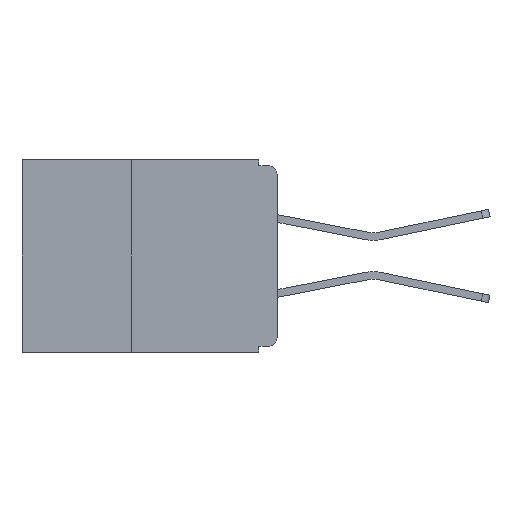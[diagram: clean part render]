
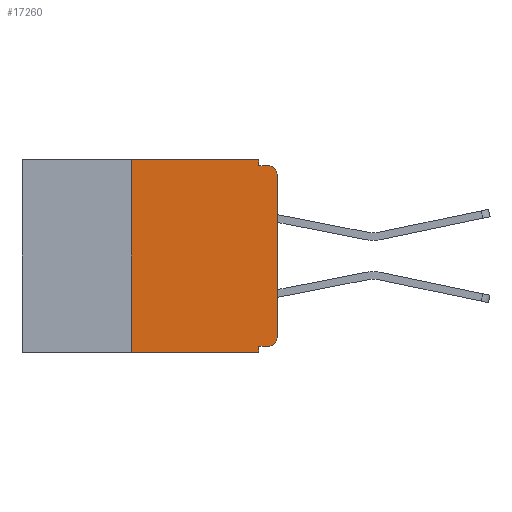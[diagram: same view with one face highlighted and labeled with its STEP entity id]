
A CAD part, left-side view. The second image highlights one B-rep face of the part: STEP entity #17260.
In plain terms, the highlighted planar face has unit normal (-1, 0, 0).
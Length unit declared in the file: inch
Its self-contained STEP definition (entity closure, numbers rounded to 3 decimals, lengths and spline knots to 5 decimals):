
#259 = CARTESIAN_POINT ( 'NONE',  ( 0., 0., -0.305 ) ) ;
#362 = CARTESIAN_POINT ( 'NONE',  ( 0., 0.015, -0.305 ) ) ;
#525 = LINE ( 'NONE', #21189, #6271 ) ;
#812 = CIRCLE ( 'NONE', #27295, 0.015 ) ;
#1344 = ORIENTED_EDGE ( 'NONE', *, *, #1648, .F. ) ;
#1469 = ORIENTED_EDGE ( 'NONE', *, *, #7640, .F. ) ;
#1493 = AXIS2_PLACEMENT_3D ( 'NONE', #25879, #11175, #28337 ) ;
#1648 = EDGE_CURVE ( 'NONE', #16640, #24566, #22728, .T. ) ;
#1978 = EDGE_CURVE ( 'NONE', #24566, #7987, #525, .T. ) ;
#2116 = CARTESIAN_POINT ( 'NONE',  ( 0., 0.25, -0.33 ) ) ;
#2266 = DIRECTION ( 'NONE',  ( 0., 0., -1. ) ) ;
#2871 = DIRECTION ( 'NONE',  ( 0., 0., -1. ) ) ;
#3144 = LINE ( 'NONE', #5762, #28352 ) ;
#4116 = CARTESIAN_POINT ( 'NONE',  ( 0., 0.25, 0. ) ) ;
#5068 = ORIENTED_EDGE ( 'NONE', *, *, #12646, .T. ) ;
#5255 = VERTEX_POINT ( 'NONE', #22413 ) ;
#5286 = VECTOR ( 'NONE', #30228, 39.37008 ) ;
#5336 = ORIENTED_EDGE ( 'NONE', *, *, #23204, .F. ) ;
#5560 = CARTESIAN_POINT ( 'NONE',  ( 0., 0.031, 0. ) ) ;
#5762 = CARTESIAN_POINT ( 'NONE',  ( 0., 0.437, -0.33 ) ) ;
#6271 = VECTOR ( 'NONE', #25772, 39.37008 ) ;
#7194 = CARTESIAN_POINT ( 'NONE',  ( 0., 0., -0.025 ) ) ;
#7640 = EDGE_CURVE ( 'NONE', #5255, #25740, #27625, .T. ) ;
#7987 = VERTEX_POINT ( 'NONE', #16604 ) ;
#8004 = DIRECTION ( 'NONE',  ( 0., -1., 0. ) ) ;
#8233 = ORIENTED_EDGE ( 'NONE', *, *, #10776, .F. ) ;
#9133 = CARTESIAN_POINT ( 'NONE',  ( 0., 0., 0. ) ) ;
#10000 = VERTEX_POINT ( 'NONE', #14814 ) ;
#10196 = ORIENTED_EDGE ( 'NONE', *, *, #29109, .T. ) ;
#10197 = VERTEX_POINT ( 'NONE', #20509 ) ;
#10776 = EDGE_CURVE ( 'NONE', #7987, #5255, #10819, .T. ) ;
#10819 = LINE ( 'NONE', #5560, #17305 ) ;
#11124 = EDGE_CURVE ( 'NONE', #14362, #25416, #14579, .T. ) ;
#11175 = DIRECTION ( 'NONE',  ( -1., 0., 0. ) ) ;
#11578 = DIRECTION ( 'NONE',  ( 0., 0., 1. ) ) ;
#11841 = DIRECTION ( 'NONE',  ( 1., 0., 0. ) ) ;
#12646 = EDGE_CURVE ( 'NONE', #10197, #14362, #812, .T. ) ;
#13356 = CARTESIAN_POINT ( 'NONE',  ( 0., 0.015, -0.01 ) ) ;
#13827 = VECTOR ( 'NONE', #11578, 39.37008 ) ;
#14362 = VERTEX_POINT ( 'NONE', #259 ) ;
#14579 = LINE ( 'NONE', #9133, #13827 ) ;
#14760 = LINE ( 'NONE', #27807, #5286 ) ;
#14814 = CARTESIAN_POINT ( 'NONE',  ( 0., 0.031, -0.33 ) ) ;
#15218 = AXIS2_PLACEMENT_3D ( 'NONE', #26538, #11841, #28987 ) ;
#15397 = VECTOR ( 'NONE', #30156, 39.37008 ) ;
#16330 = LINE ( 'NONE', #31519, #28626 ) ;
#16604 = CARTESIAN_POINT ( 'NONE',  ( 0., 0.031, 0. ) ) ;
#16640 = VERTEX_POINT ( 'NONE', #2116 ) ;
#17260 = ADVANCED_FACE ( 'NONE', ( #31479 ), #19121, .F. ) ;
#17305 = VECTOR ( 'NONE', #27472, 39.37008 ) ;
#17426 = DIRECTION ( 'NONE',  ( -1., 0., 0. ) ) ;
#19121 = PLANE ( 'NONE',  #15218 ) ;
#19255 = ORIENTED_EDGE ( 'NONE', *, *, #21165, .T. ) ;
#20031 = EDGE_LOOP ( 'NONE', ( #29079, #19255, #1469, #8233, #29008, #1344, #10196, #5336, #28726, #5068 ) ) ;
#20509 = CARTESIAN_POINT ( 'NONE',  ( 0., 0.015, -0.32 ) ) ;
#21064 = EDGE_CURVE ( 'NONE', #10197, #22748, #14760, .T. ) ;
#21165 = EDGE_CURVE ( 'NONE', #25416, #25740, #21679, .T. ) ;
#21189 = CARTESIAN_POINT ( 'NONE',  ( 0., 0.437, 0. ) ) ;
#21679 = CIRCLE ( 'NONE', #1493, 0.015 ) ;
#22413 = CARTESIAN_POINT ( 'NONE',  ( 0., 0.031, -0.01 ) ) ;
#22445 = CARTESIAN_POINT ( 'NONE',  ( 0., 0.031, -0.32 ) ) ;
#22728 = LINE ( 'NONE', #30080, #15397 ) ;
#22748 = VERTEX_POINT ( 'NONE', #22445 ) ;
#22843 = DIRECTION ( 'NONE',  ( 0., -1., 0. ) ) ;
#23204 = EDGE_CURVE ( 'NONE', #22748, #10000, #16330, .T. ) ;
#24566 = VERTEX_POINT ( 'NONE', #4116 ) ;
#25416 = VERTEX_POINT ( 'NONE', #7194 ) ;
#25740 = VERTEX_POINT ( 'NONE', #13356 ) ;
#25772 = DIRECTION ( 'NONE',  ( 0., -1., 0. ) ) ;
#25879 = CARTESIAN_POINT ( 'NONE',  ( 0., 0.015, -0.025 ) ) ;
#26538 = CARTESIAN_POINT ( 'NONE',  ( 0., 0.437, 0. ) ) ;
#26865 = VECTOR ( 'NONE', #8004, 39.37008 ) ;
#27295 = AXIS2_PLACEMENT_3D ( 'NONE', #362, #17426, #2871 ) ;
#27472 = DIRECTION ( 'NONE',  ( 0., 0., -1. ) ) ;
#27598 = CARTESIAN_POINT ( 'NONE',  ( 0., 0., -0.01 ) ) ;
#27625 = LINE ( 'NONE', #27598, #26865 ) ;
#27807 = CARTESIAN_POINT ( 'NONE',  ( 0., 0., -0.32 ) ) ;
#28337 = DIRECTION ( 'NONE',  ( 0., 0., -1. ) ) ;
#28352 = VECTOR ( 'NONE', #22843, 39.37008 ) ;
#28626 = VECTOR ( 'NONE', #2266, 39.37008 ) ;
#28726 = ORIENTED_EDGE ( 'NONE', *, *, #21064, .F. ) ;
#28987 = DIRECTION ( 'NONE',  ( 0., 0., -1. ) ) ;
#29008 = ORIENTED_EDGE ( 'NONE', *, *, #1978, .F. ) ;
#29079 = ORIENTED_EDGE ( 'NONE', *, *, #11124, .T. ) ;
#29109 = EDGE_CURVE ( 'NONE', #16640, #10000, #3144, .T. ) ;
#30080 = CARTESIAN_POINT ( 'NONE',  ( 0., 0.25, -0.33 ) ) ;
#30156 = DIRECTION ( 'NONE',  ( 0., 0., 1. ) ) ;
#30228 = DIRECTION ( 'NONE',  ( 0., 1., 0. ) ) ;
#31479 = FACE_OUTER_BOUND ( 'NONE', #20031, .T. ) ;
#31519 = CARTESIAN_POINT ( 'NONE',  ( 0., 0.031, -0.33 ) ) ;
